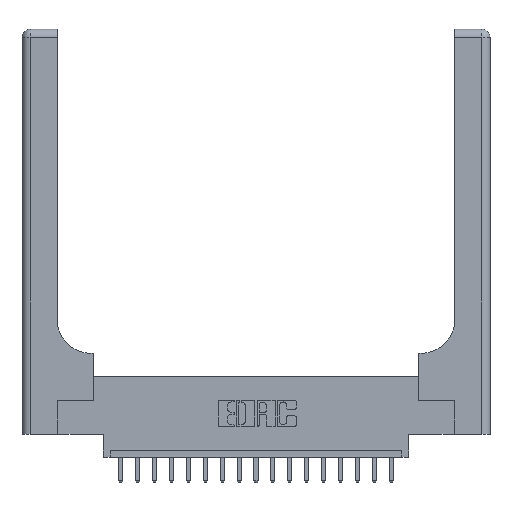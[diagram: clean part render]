
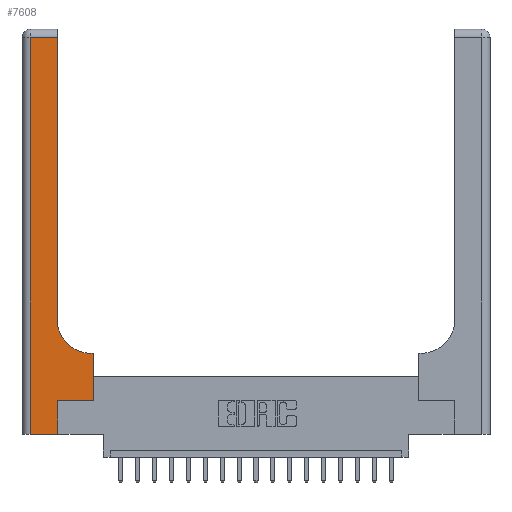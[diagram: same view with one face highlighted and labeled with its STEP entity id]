
A CAD part, top view. The second image highlights one B-rep face of the part: STEP entity #7608.
In plain terms, the highlighted planar face has unit normal (0, 0, 1).
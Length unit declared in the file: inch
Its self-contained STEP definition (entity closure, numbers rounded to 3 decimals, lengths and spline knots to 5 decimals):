
#840 = CARTESIAN_POINT ( 'NONE',  ( 0.26, 0.85, 0.37 ) ) ;
#919 = CARTESIAN_POINT ( 'NONE',  ( 0.26, 0.6, 0.37 ) ) ;
#1063 = VERTEX_POINT ( 'NONE', #840 ) ;
#1221 = CARTESIAN_POINT ( 'NONE',  ( 0.06, 3., 0.37 ) ) ;
#1243 = CARTESIAN_POINT ( 'NONE',  ( 0., 0., 0.37 ) ) ;
#1350 = VECTOR ( 'NONE', #7313, 39.37008 ) ;
#1408 = EDGE_LOOP ( 'NONE', ( #18512, #1768, #7756, #16985, #15904, #4064, #7703, #15364, #9794 ) ) ;
#1444 = DIRECTION ( 'NONE',  ( 1., 0., 0. ) ) ;
#1768 = ORIENTED_EDGE ( 'NONE', *, *, #7306, .T. ) ;
#2597 = DIRECTION ( 'NONE',  ( -1., 0., 0. ) ) ;
#2652 = CARTESIAN_POINT ( 'NONE',  ( 0.265, 0., 0.37 ) ) ;
#2718 = LINE ( 'NONE', #1221, #1350 ) ;
#2743 = CARTESIAN_POINT ( 'NONE',  ( 0.51, 0.85, 0.37 ) ) ;
#2773 = EDGE_CURVE ( 'NONE', #11290, #9944, #12939, .T. ) ;
#2948 = VECTOR ( 'NONE', #5321, 39.37008 ) ;
#3292 = VECTOR ( 'NONE', #17347, 39.37008 ) ;
#4028 = CARTESIAN_POINT ( 'NONE',  ( 0.528, 0.6, 0.37 ) ) ;
#4064 = ORIENTED_EDGE ( 'NONE', *, *, #14951, .T. ) ;
#4185 = AXIS2_PLACEMENT_3D ( 'NONE', #12411, #15694, #7892 ) ;
#4237 = EDGE_CURVE ( 'NONE', #15385, #12179, #2718, .T. ) ;
#4549 = EDGE_CURVE ( 'NONE', #6675, #11290, #19514, .T. ) ;
#5321 = DIRECTION ( 'NONE',  ( -1., 0., 0. ) ) ;
#5900 = CARTESIAN_POINT ( 'NONE',  ( 0.528, 0.25, 0.37 ) ) ;
#6159 = VECTOR ( 'NONE', #12014, 39.37008 ) ;
#6547 = CARTESIAN_POINT ( 'NONE',  ( 0.06, 0., 0.37 ) ) ;
#6675 = VERTEX_POINT ( 'NONE', #16649 ) ;
#7306 = EDGE_CURVE ( 'NONE', #7568, #15385, #8703, .T. ) ;
#7313 = DIRECTION ( 'NONE',  ( 0., -1., 0. ) ) ;
#7568 = VERTEX_POINT ( 'NONE', #11300 ) ;
#7608 = ADVANCED_FACE ( 'NONE', ( #10900 ), #16998, .F. ) ;
#7703 = ORIENTED_EDGE ( 'NONE', *, *, #4549, .T. ) ;
#7756 = ORIENTED_EDGE ( 'NONE', *, *, #4237, .T. ) ;
#7799 = CIRCLE ( 'NONE', #13883, 0.25 ) ;
#7892 = DIRECTION ( 'NONE',  ( -1., 0., 0. ) ) ;
#8128 = EDGE_CURVE ( 'NONE', #11039, #12169, #17247, .T. ) ;
#8144 = CARTESIAN_POINT ( 'NONE',  ( 0.265, 0., 0.37 ) ) ;
#8703 = LINE ( 'NONE', #14912, #13271 ) ;
#8785 = VECTOR ( 'NONE', #10654, 39.37008 ) ;
#8864 = VECTOR ( 'NONE', #19024, 39.37008 ) ;
#9049 = LINE ( 'NONE', #1243, #11101 ) ;
#9247 = CARTESIAN_POINT ( 'NONE',  ( 0.26, 3., 0.37 ) ) ;
#9548 = CARTESIAN_POINT ( 'NONE',  ( 0.265, 0.25, 0.37 ) ) ;
#9697 = EDGE_CURVE ( 'NONE', #9944, #1063, #7799, .T. ) ;
#9794 = ORIENTED_EDGE ( 'NONE', *, *, #9697, .T. ) ;
#9944 = VERTEX_POINT ( 'NONE', #16756 ) ;
#9946 = EDGE_CURVE ( 'NONE', #1063, #7568, #18658, .T. ) ;
#10654 = DIRECTION ( 'NONE',  ( 0., 1., 0. ) ) ;
#10900 = FACE_OUTER_BOUND ( 'NONE', #1408, .T. ) ;
#11039 = VERTEX_POINT ( 'NONE', #2652 ) ;
#11101 = VECTOR ( 'NONE', #1444, 39.37008 ) ;
#11290 = VERTEX_POINT ( 'NONE', #4028 ) ;
#11300 = CARTESIAN_POINT ( 'NONE',  ( 0.26, 2.94, 0.37 ) ) ;
#11766 = DIRECTION ( 'NONE',  ( 1., 0., 0. ) ) ;
#12014 = DIRECTION ( 'NONE',  ( 0., 1., 0. ) ) ;
#12169 = VERTEX_POINT ( 'NONE', #9548 ) ;
#12179 = VERTEX_POINT ( 'NONE', #6547 ) ;
#12411 = CARTESIAN_POINT ( 'NONE',  ( 0., 3., 0.37 ) ) ;
#12921 = CARTESIAN_POINT ( 'NONE',  ( 0.265, 0.25, 0.37 ) ) ;
#12939 = LINE ( 'NONE', #919, #2948 ) ;
#13271 = VECTOR ( 'NONE', #2597, 39.37008 ) ;
#13883 = AXIS2_PLACEMENT_3D ( 'NONE', #2743, #19468, #11766 ) ;
#14390 = CARTESIAN_POINT ( 'NONE',  ( 0.06, 2.94, 0.37 ) ) ;
#14664 = EDGE_CURVE ( 'NONE', #12179, #11039, #9049, .T. ) ;
#14912 = CARTESIAN_POINT ( 'NONE',  ( 0., 2.94, 0.37 ) ) ;
#14951 = EDGE_CURVE ( 'NONE', #12169, #6675, #15909, .T. ) ;
#15364 = ORIENTED_EDGE ( 'NONE', *, *, #2773, .T. ) ;
#15385 = VERTEX_POINT ( 'NONE', #14390 ) ;
#15694 = DIRECTION ( 'NONE',  ( 0., 0., -1. ) ) ;
#15904 = ORIENTED_EDGE ( 'NONE', *, *, #8128, .T. ) ;
#15909 = LINE ( 'NONE', #12921, #8864 ) ;
#16649 = CARTESIAN_POINT ( 'NONE',  ( 0.528, 0.25, 0.37 ) ) ;
#16756 = CARTESIAN_POINT ( 'NONE',  ( 0.51, 0.6, 0.37 ) ) ;
#16985 = ORIENTED_EDGE ( 'NONE', *, *, #14664, .T. ) ;
#16998 = PLANE ( 'NONE',  #4185 ) ;
#17247 = LINE ( 'NONE', #8144, #3292 ) ;
#17347 = DIRECTION ( 'NONE',  ( 0., 1., 0. ) ) ;
#18512 = ORIENTED_EDGE ( 'NONE', *, *, #9946, .T. ) ;
#18658 = LINE ( 'NONE', #9247, #8785 ) ;
#19024 = DIRECTION ( 'NONE',  ( 1., 0., 0. ) ) ;
#19468 = DIRECTION ( 'NONE',  ( 0., 0., -1. ) ) ;
#19514 = LINE ( 'NONE', #5900, #6159 ) ;
